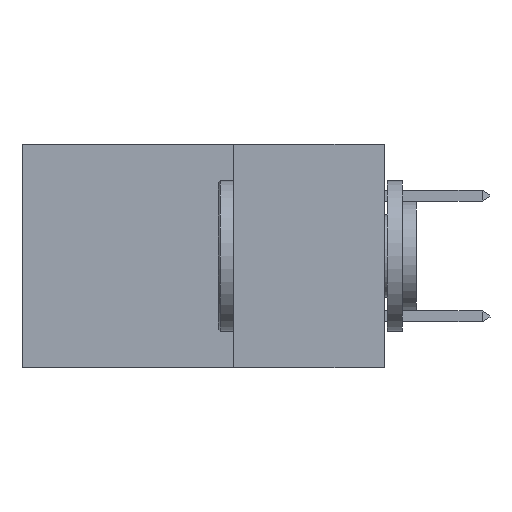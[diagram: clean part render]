
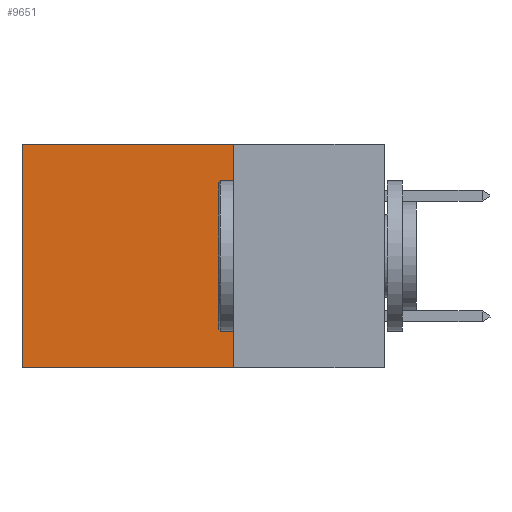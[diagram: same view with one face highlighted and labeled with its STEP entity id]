
A CAD part, left-side view. The second image highlights one B-rep face of the part: STEP entity #9651.
In plain terms, the highlighted planar face has unit normal (-1, 0, 0).
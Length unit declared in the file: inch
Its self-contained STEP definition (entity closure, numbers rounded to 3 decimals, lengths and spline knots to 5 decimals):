
#810 = ORIENTED_EDGE ( 'NONE', *, *, #13909, .T. ) ;
#1019 = DIRECTION ( 'NONE',  ( 0., 0., -1. ) ) ;
#1297 = EDGE_CURVE ( 'NONE', #18301, #21349, #12572, .T. ) ;
#1882 = EDGE_CURVE ( 'NONE', #20048, #21349, #9174, .T. ) ;
#4754 = VERTEX_POINT ( 'NONE', #19607 ) ;
#6457 = CARTESIAN_POINT ( 'NONE',  ( 0.2875, 0.6, 0. ) ) ;
#8642 = CARTESIAN_POINT ( 'NONE',  ( 0.2875, 0.25, 0. ) ) ;
#9174 = LINE ( 'NONE', #12340, #13869 ) ;
#9312 = LINE ( 'NONE', #8642, #14011 ) ;
#9651 = ADVANCED_FACE ( 'NONE', ( #17032 ), #21846, .F. ) ;
#11463 = DIRECTION ( 'NONE',  ( 1., 0., 0. ) ) ;
#12282 = DIRECTION ( 'NONE',  ( 0., 0., -1. ) ) ;
#12340 = CARTESIAN_POINT ( 'NONE',  ( 0.2875, 0.6, 0. ) ) ;
#12572 = LINE ( 'NONE', #14955, #16701 ) ;
#12801 = AXIS2_PLACEMENT_3D ( 'NONE', #14988, #11463, #1019 ) ;
#13115 = CARTESIAN_POINT ( 'NONE',  ( 0.2875, 0.25, 0. ) ) ;
#13795 = DIRECTION ( 'NONE',  ( 0., 1., 0. ) ) ;
#13852 = EDGE_LOOP ( 'NONE', ( #19976, #19688, #18471, #810 ) ) ;
#13869 = VECTOR ( 'NONE', #12282, 39.37008 ) ;
#13909 = EDGE_CURVE ( 'NONE', #4754, #20048, #9312, .T. ) ;
#14011 = VECTOR ( 'NONE', #15559, 39.37008 ) ;
#14955 = CARTESIAN_POINT ( 'NONE',  ( 0.2875, 0.25, -0.37 ) ) ;
#14988 = CARTESIAN_POINT ( 'NONE',  ( 0.2875, 0.25, 0. ) ) ;
#15559 = DIRECTION ( 'NONE',  ( 0., 1., 0. ) ) ;
#16598 = DIRECTION ( 'NONE',  ( 0., 0., -1. ) ) ;
#16701 = VECTOR ( 'NONE', #13795, 39.37008 ) ;
#17032 = FACE_OUTER_BOUND ( 'NONE', #13852, .T. ) ;
#17244 = CARTESIAN_POINT ( 'NONE',  ( 0.2875, 0.25, -0.37 ) ) ;
#17309 = EDGE_CURVE ( 'NONE', #4754, #18301, #21092, .T. ) ;
#18301 = VERTEX_POINT ( 'NONE', #17244 ) ;
#18471 = ORIENTED_EDGE ( 'NONE', *, *, #17309, .F. ) ;
#19607 = CARTESIAN_POINT ( 'NONE',  ( 0.2875, 0.25, 0. ) ) ;
#19688 = ORIENTED_EDGE ( 'NONE', *, *, #1297, .F. ) ;
#19976 = ORIENTED_EDGE ( 'NONE', *, *, #1882, .T. ) ;
#20048 = VERTEX_POINT ( 'NONE', #6457 ) ;
#21092 = LINE ( 'NONE', #13115, #22104 ) ;
#21349 = VERTEX_POINT ( 'NONE', #21639 ) ;
#21639 = CARTESIAN_POINT ( 'NONE',  ( 0.2875, 0.6, -0.37 ) ) ;
#21846 = PLANE ( 'NONE',  #12801 ) ;
#22104 = VECTOR ( 'NONE', #16598, 39.37008 ) ;
